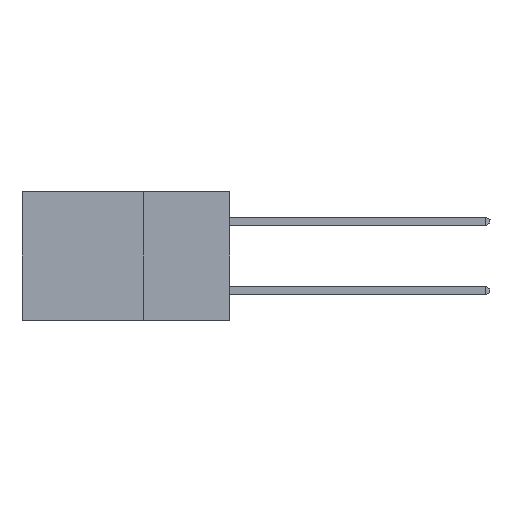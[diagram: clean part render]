
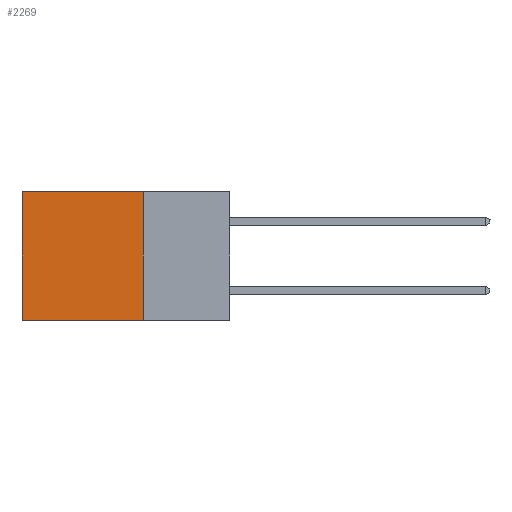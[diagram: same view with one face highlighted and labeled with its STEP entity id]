
A CAD part, left-side view. The second image highlights one B-rep face of the part: STEP entity #2269.
In plain terms, the highlighted planar face has unit normal (-1, 0, 0).
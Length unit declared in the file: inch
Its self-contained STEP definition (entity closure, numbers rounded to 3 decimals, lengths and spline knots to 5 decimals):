
#13 = AXIS2_PLACEMENT_3D ( 'NONE', #7686, #4753, #1917 ) ;
#1052 = VECTOR ( 'NONE', #5304, 39.37008 ) ;
#1917 = DIRECTION ( 'NONE',  ( 0., 0., -1. ) ) ;
#1983 = VERTEX_POINT ( 'NONE', #11774 ) ;
#2269 = ADVANCED_FACE ( 'NONE', ( #3770 ), #10509, .F. ) ;
#3213 = DIRECTION ( 'NONE',  ( 0., 1., 0. ) ) ;
#3770 = FACE_OUTER_BOUND ( 'NONE', #4269, .T. ) ;
#4189 = VECTOR ( 'NONE', #3213, 39.37008 ) ;
#4259 = VECTOR ( 'NONE', #9852, 39.37008 ) ;
#4269 = EDGE_LOOP ( 'NONE', ( #5709, #4942, #10358, #5236 ) ) ;
#4292 = EDGE_CURVE ( 'NONE', #6616, #7992, #9436, .T. ) ;
#4332 = CARTESIAN_POINT ( 'NONE',  ( 0.298, 0.25, 0. ) ) ;
#4753 = DIRECTION ( 'NONE',  ( 1., 0., 0. ) ) ;
#4942 = ORIENTED_EDGE ( 'NONE', *, *, #4292, .F. ) ;
#5236 = ORIENTED_EDGE ( 'NONE', *, *, #9583, .T. ) ;
#5304 = DIRECTION ( 'NONE',  ( 0., 1., 0. ) ) ;
#5709 = ORIENTED_EDGE ( 'NONE', *, *, #5874, .T. ) ;
#5874 = EDGE_CURVE ( 'NONE', #11553, #7992, #8666, .T. ) ;
#5918 = LINE ( 'NONE', #10774, #4259 ) ;
#6206 = CARTESIAN_POINT ( 'NONE',  ( 0.298, 0.6, 0. ) ) ;
#6274 = VECTOR ( 'NONE', #7024, 39.37008 ) ;
#6616 = VERTEX_POINT ( 'NONE', #12425 ) ;
#7024 = DIRECTION ( 'NONE',  ( 0., 0., -1. ) ) ;
#7686 = CARTESIAN_POINT ( 'NONE',  ( 0.298, 0.25, 0. ) ) ;
#7992 = VERTEX_POINT ( 'NONE', #10406 ) ;
#8100 = EDGE_CURVE ( 'NONE', #1983, #6616, #5918, .T. ) ;
#8666 = LINE ( 'NONE', #10840, #6274 ) ;
#9436 = LINE ( 'NONE', #11869, #4189 ) ;
#9583 = EDGE_CURVE ( 'NONE', #1983, #11553, #10685, .T. ) ;
#9852 = DIRECTION ( 'NONE',  ( 0., 0., -1. ) ) ;
#10358 = ORIENTED_EDGE ( 'NONE', *, *, #8100, .F. ) ;
#10406 = CARTESIAN_POINT ( 'NONE',  ( 0.298, 0.6, -0.37 ) ) ;
#10509 = PLANE ( 'NONE',  #13 ) ;
#10685 = LINE ( 'NONE', #4332, #1052 ) ;
#10774 = CARTESIAN_POINT ( 'NONE',  ( 0.298, 0.25, 0. ) ) ;
#10840 = CARTESIAN_POINT ( 'NONE',  ( 0.298, 0.6, 0. ) ) ;
#11553 = VERTEX_POINT ( 'NONE', #6206 ) ;
#11774 = CARTESIAN_POINT ( 'NONE',  ( 0.298, 0.25, 0. ) ) ;
#11869 = CARTESIAN_POINT ( 'NONE',  ( 0.298, 0.25, -0.37 ) ) ;
#12425 = CARTESIAN_POINT ( 'NONE',  ( 0.298, 0.25, -0.37 ) ) ;
